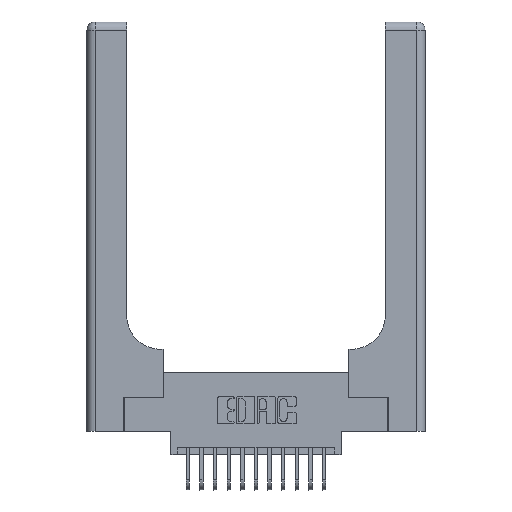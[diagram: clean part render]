
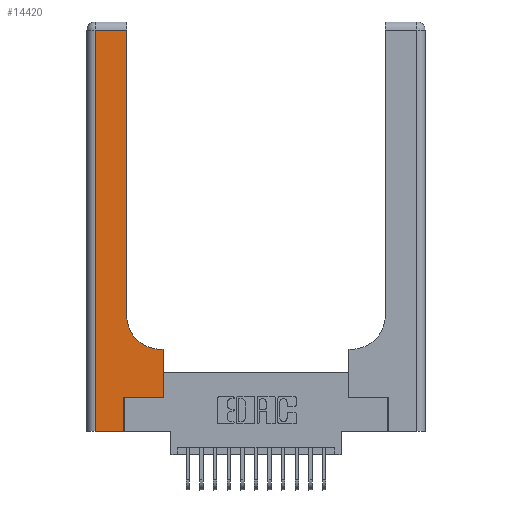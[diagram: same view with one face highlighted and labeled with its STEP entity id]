
A CAD part, top view. The second image highlights one B-rep face of the part: STEP entity #14420.
In plain terms, the highlighted planar face has unit normal (0, 0, 1).
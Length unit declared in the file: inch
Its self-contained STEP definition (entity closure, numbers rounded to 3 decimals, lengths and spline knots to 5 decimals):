
#45 = VERTEX_POINT ( 'NONE', #1921 ) ;
#249 = ORIENTED_EDGE ( 'NONE', *, *, #10498, .T. ) ;
#330 = VERTEX_POINT ( 'NONE', #7305 ) ;
#338 = VERTEX_POINT ( 'NONE', #10440 ) ;
#374 = DIRECTION ( 'NONE',  ( 0., 0., -1. ) ) ;
#877 = DIRECTION ( 'NONE',  ( -1., 0., 0. ) ) ;
#1070 = DIRECTION ( 'NONE',  ( 0., 0., -1. ) ) ;
#1488 = ORIENTED_EDGE ( 'NONE', *, *, #8166, .T. ) ;
#1921 = CARTESIAN_POINT ( 'NONE',  ( 0.2915, 2.94, 0.37 ) ) ;
#2236 = VECTOR ( 'NONE', #9019, 39.37008 ) ;
#2747 = VERTEX_POINT ( 'NONE', #13355 ) ;
#2879 = EDGE_CURVE ( 'NONE', #15012, #45, #15642, .T. ) ;
#3163 = DIRECTION ( 'NONE',  ( -1., 0., 0. ) ) ;
#3270 = CARTESIAN_POINT ( 'NONE',  ( 0.269, 0.25, 0.37 ) ) ;
#4917 = CIRCLE ( 'NONE', #17997, 0.25 ) ;
#4923 = EDGE_CURVE ( 'NONE', #18211, #13305, #13587, .T. ) ;
#5454 = VECTOR ( 'NONE', #10883, 39.37008 ) ;
#5523 = CARTESIAN_POINT ( 'NONE',  ( 0., 3., 0.37 ) ) ;
#5556 = EDGE_CURVE ( 'NONE', #13305, #18990, #18164, .T. ) ;
#5613 = LINE ( 'NONE', #3270, #15689 ) ;
#5837 = VECTOR ( 'NONE', #10753, 39.37008 ) ;
#5873 = CARTESIAN_POINT ( 'NONE',  ( 0.269, 0., 0.37 ) ) ;
#6326 = LINE ( 'NONE', #5873, #5837 ) ;
#6480 = DIRECTION ( 'NONE',  ( 1., 0., 0. ) ) ;
#6551 = EDGE_CURVE ( 'NONE', #18990, #15012, #4917, .T. ) ;
#6867 = CARTESIAN_POINT ( 'NONE',  ( 0.06, 3., 0.37 ) ) ;
#6934 = CARTESIAN_POINT ( 'NONE',  ( 0., 2.94, 0.37 ) ) ;
#7084 = VECTOR ( 'NONE', #17789, 39.37008 ) ;
#7305 = CARTESIAN_POINT ( 'NONE',  ( 0.269, 0., 0.37 ) ) ;
#7331 = EDGE_CURVE ( 'NONE', #2747, #338, #12600, .T. ) ;
#7402 = EDGE_CURVE ( 'NONE', #45, #2747, #14028, .T. ) ;
#8004 = CARTESIAN_POINT ( 'NONE',  ( 0.5585, 0.25, 0.37 ) ) ;
#8166 = EDGE_CURVE ( 'NONE', #12557, #18211, #5613, .T. ) ;
#8197 = CARTESIAN_POINT ( 'NONE',  ( 0.5415, 0.6, 0.37 ) ) ;
#8520 = VECTOR ( 'NONE', #14679, 39.37008 ) ;
#8571 = EDGE_CURVE ( 'NONE', #338, #330, #18794, .T. ) ;
#8823 = DIRECTION ( 'NONE',  ( 1., 0., 0. ) ) ;
#8859 = ORIENTED_EDGE ( 'NONE', *, *, #7331, .T. ) ;
#8884 = CARTESIAN_POINT ( 'NONE',  ( 0., 0., 0.37 ) ) ;
#9019 = DIRECTION ( 'NONE',  ( 0., 1., 0. ) ) ;
#9035 = VECTOR ( 'NONE', #3163, 39.37008 ) ;
#9063 = ORIENTED_EDGE ( 'NONE', *, *, #7402, .T. ) ;
#10440 = CARTESIAN_POINT ( 'NONE',  ( 0.06, 0., 0.37 ) ) ;
#10498 = EDGE_CURVE ( 'NONE', #330, #12557, #6326, .T. ) ;
#10753 = DIRECTION ( 'NONE',  ( 0., 1., 0. ) ) ;
#10883 = DIRECTION ( 'NONE',  ( 0., 1., 0. ) ) ;
#11034 = ORIENTED_EDGE ( 'NONE', *, *, #4923, .T. ) ;
#11921 = FACE_OUTER_BOUND ( 'NONE', #18864, .T. ) ;
#11998 = ORIENTED_EDGE ( 'NONE', *, *, #6551, .T. ) ;
#12066 = CARTESIAN_POINT ( 'NONE',  ( 0.2915, 0.6, 0.37 ) ) ;
#12557 = VERTEX_POINT ( 'NONE', #18316 ) ;
#12600 = LINE ( 'NONE', #6867, #7084 ) ;
#13004 = VECTOR ( 'NONE', #8823, 39.37008 ) ;
#13083 = PLANE ( 'NONE',  #18935 ) ;
#13205 = ORIENTED_EDGE ( 'NONE', *, *, #2879, .T. ) ;
#13305 = VERTEX_POINT ( 'NONE', #18161 ) ;
#13355 = CARTESIAN_POINT ( 'NONE',  ( 0.06, 2.94, 0.37 ) ) ;
#13587 = LINE ( 'NONE', #8004, #5454 ) ;
#14028 = LINE ( 'NONE', #6934, #8520 ) ;
#14420 = ADVANCED_FACE ( 'NONE', ( #11921 ), #13083, .F. ) ;
#14679 = DIRECTION ( 'NONE',  ( -1., 0., 0. ) ) ;
#14685 = ORIENTED_EDGE ( 'NONE', *, *, #5556, .T. ) ;
#15012 = VERTEX_POINT ( 'NONE', #18785 ) ;
#15293 = ORIENTED_EDGE ( 'NONE', *, *, #8571, .T. ) ;
#15642 = LINE ( 'NONE', #18283, #2236 ) ;
#15689 = VECTOR ( 'NONE', #6480, 39.37008 ) ;
#15820 = CARTESIAN_POINT ( 'NONE',  ( 0.5585, 0.25, 0.37 ) ) ;
#17423 = CARTESIAN_POINT ( 'NONE',  ( 0.5415, 0.85, 0.37 ) ) ;
#17789 = DIRECTION ( 'NONE',  ( 0., -1., 0. ) ) ;
#17997 = AXIS2_PLACEMENT_3D ( 'NONE', #17423, #374, #18959 ) ;
#18161 = CARTESIAN_POINT ( 'NONE',  ( 0.5585, 0.6, 0.37 ) ) ;
#18164 = LINE ( 'NONE', #12066, #9035 ) ;
#18211 = VERTEX_POINT ( 'NONE', #15820 ) ;
#18283 = CARTESIAN_POINT ( 'NONE',  ( 0.2915, 3., 0.37 ) ) ;
#18316 = CARTESIAN_POINT ( 'NONE',  ( 0.269, 0.25, 0.37 ) ) ;
#18785 = CARTESIAN_POINT ( 'NONE',  ( 0.2915, 0.85, 0.37 ) ) ;
#18794 = LINE ( 'NONE', #8884, #13004 ) ;
#18864 = EDGE_LOOP ( 'NONE', ( #13205, #9063, #8859, #15293, #249, #1488, #11034, #14685, #11998 ) ) ;
#18935 = AXIS2_PLACEMENT_3D ( 'NONE', #5523, #1070, #877 ) ;
#18959 = DIRECTION ( 'NONE',  ( 1., 0., 0. ) ) ;
#18990 = VERTEX_POINT ( 'NONE', #8197 ) ;
